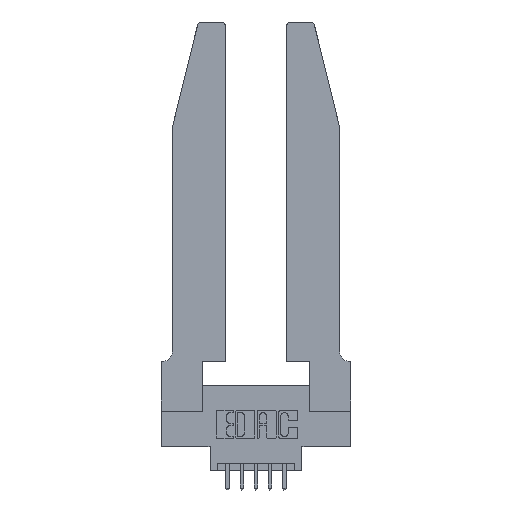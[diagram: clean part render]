
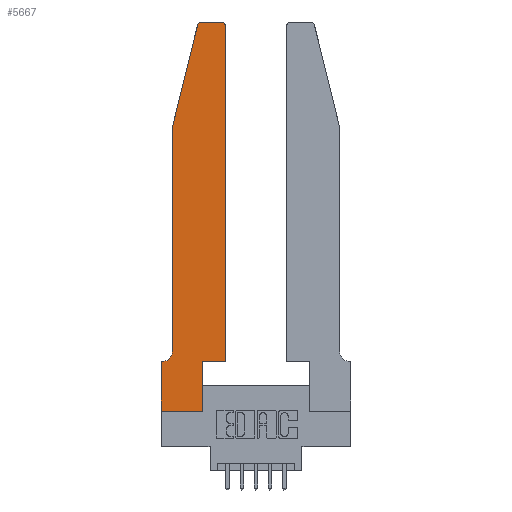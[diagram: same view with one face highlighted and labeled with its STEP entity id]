
A CAD part, top view. The second image highlights one B-rep face of the part: STEP entity #5667.
In plain terms, the highlighted planar face has unit normal (0, 0, 1).
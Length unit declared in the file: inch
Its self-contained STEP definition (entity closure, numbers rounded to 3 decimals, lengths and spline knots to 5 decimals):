
#4 = DIRECTION ( 'NONE',  ( 1., 0., 0. ) ) ;
#141 = VECTOR ( 'NONE', #9166, 39.37008 ) ;
#238 = LINE ( 'NONE', #2902, #11358 ) ;
#588 = CARTESIAN_POINT ( 'NONE',  ( 0.0755, 0.35, 0.37 ) ) ;
#594 = ORIENTED_EDGE ( 'NONE', *, *, #11141, .T. ) ;
#834 = DIRECTION ( 'NONE',  ( -1., 0., 0. ) ) ;
#885 = VERTEX_POINT ( 'NONE', #13201 ) ;
#962 = ORIENTED_EDGE ( 'NONE', *, *, #2790, .T. ) ;
#1181 = AXIS2_PLACEMENT_3D ( 'NONE', #13568, #7385, #834 ) ;
#1326 = DIRECTION ( 'NONE',  ( 0., 0., 1. ) ) ;
#1408 = ORIENTED_EDGE ( 'NONE', *, *, #4355, .T. ) ;
#1425 = DIRECTION ( 'NONE',  ( 0., -1., 0. ) ) ;
#1457 = LINE ( 'NONE', #11783, #10041 ) ;
#1467 = CARTESIAN_POINT ( 'NONE',  ( 0.0755, 2., 0.37 ) ) ;
#1706 = DIRECTION ( 'NONE',  ( 1., 0., 0. ) ) ;
#1748 = CARTESIAN_POINT ( 'NONE',  ( 0.2865, 0.35, 0.37 ) ) ;
#1940 = VECTOR ( 'NONE', #13599, 39.37008 ) ;
#2302 = ORIENTED_EDGE ( 'NONE', *, *, #7899, .T. ) ;
#2636 = ORIENTED_EDGE ( 'NONE', *, *, #11232, .T. ) ;
#2716 = EDGE_LOOP ( 'NONE', ( #1408, #4652, #2302, #10080, #2636, #594, #962, #4663, #4332, #12566, #7375, #9206 ) ) ;
#2720 = CARTESIAN_POINT ( 'NONE',  ( 0., 0., 0.37 ) ) ;
#2774 = VERTEX_POINT ( 'NONE', #11372 ) ;
#2790 = EDGE_CURVE ( 'NONE', #885, #5018, #6215, .T. ) ;
#2902 = CARTESIAN_POINT ( 'NONE',  ( 0.0755, 2., 0.37 ) ) ;
#3075 = LINE ( 'NONE', #5925, #141 ) ;
#3227 = VERTEX_POINT ( 'NONE', #7248 ) ;
#3809 = CIRCLE ( 'NONE', #10134, 0.03 ) ;
#3815 = EDGE_CURVE ( 'NONE', #9651, #10955, #12226, .T. ) ;
#3924 = DIRECTION ( 'NONE',  ( -1., 0., 0. ) ) ;
#4332 = ORIENTED_EDGE ( 'NONE', *, *, #12507, .T. ) ;
#4355 = EDGE_CURVE ( 'NONE', #10137, #9304, #3075, .T. ) ;
#4362 = CARTESIAN_POINT ( 'NONE',  ( 0.2865, 0., 0.37 ) ) ;
#4652 = ORIENTED_EDGE ( 'NONE', *, *, #13527, .T. ) ;
#4663 = ORIENTED_EDGE ( 'NONE', *, *, #12418, .T. ) ;
#4891 = VECTOR ( 'NONE', #3924, 39.37008 ) ;
#4986 = CIRCLE ( 'NONE', #6332, 0.03 ) ;
#5018 = VERTEX_POINT ( 'NONE', #2720 ) ;
#5087 = DIRECTION ( 'NONE',  ( 1., 0., 0. ) ) ;
#5465 = DIRECTION ( 'NONE',  ( 0., 1., 0. ) ) ;
#5641 = VERTEX_POINT ( 'NONE', #11292 ) ;
#5667 = ADVANCED_FACE ( 'NONE', ( #5974 ), #13345, .T. ) ;
#5925 = CARTESIAN_POINT ( 'NONE',  ( 0.2605, 2.75, 0.37 ) ) ;
#5974 = FACE_OUTER_BOUND ( 'NONE', #2716, .T. ) ;
#6215 = LINE ( 'NONE', #11280, #11470 ) ;
#6226 = LINE ( 'NONE', #10391, #8732 ) ;
#6332 = AXIS2_PLACEMENT_3D ( 'NONE', #7872, #1326, #8909 ) ;
#6341 = CARTESIAN_POINT ( 'NONE',  ( 0.2865, 0.35, 0.37 ) ) ;
#6353 = DIRECTION ( 'NONE',  ( 0., 0., 1. ) ) ;
#6500 = AXIS2_PLACEMENT_3D ( 'NONE', #7137, #8232, #1706 ) ;
#6786 = CIRCLE ( 'NONE', #1181, 0.07 ) ;
#7137 = CARTESIAN_POINT ( 'NONE',  ( 0., 0.35, 0.37 ) ) ;
#7248 = CARTESIAN_POINT ( 'NONE',  ( 0.0055, 0.35, 0.37 ) ) ;
#7375 = ORIENTED_EDGE ( 'NONE', *, *, #11894, .T. ) ;
#7385 = DIRECTION ( 'NONE',  ( 0., 0., -1. ) ) ;
#7695 = CARTESIAN_POINT ( 'NONE',  ( 0.4505, 0.35, 0.37 ) ) ;
#7797 = LINE ( 'NONE', #588, #4891 ) ;
#7872 = CARTESIAN_POINT ( 'NONE',  ( 0.4205, 2.72, 0.37 ) ) ;
#7899 = EDGE_CURVE ( 'NONE', #11291, #9651, #238, .T. ) ;
#7977 = CARTESIAN_POINT ( 'NONE',  ( 0.0755, 0.42, 0.37 ) ) ;
#8232 = DIRECTION ( 'NONE',  ( 0., 0., 1. ) ) ;
#8371 = VERTEX_POINT ( 'NONE', #1748 ) ;
#8732 = VECTOR ( 'NONE', #5087, 39.37008 ) ;
#8909 = DIRECTION ( 'NONE',  ( 1., 0., 0. ) ) ;
#9166 = DIRECTION ( 'NONE',  ( -1., 0., 0. ) ) ;
#9206 = ORIENTED_EDGE ( 'NONE', *, *, #13704, .T. ) ;
#9304 = VERTEX_POINT ( 'NONE', #9733 ) ;
#9651 = VERTEX_POINT ( 'NONE', #9866 ) ;
#9733 = CARTESIAN_POINT ( 'NONE',  ( 0.284, 2.75, 0.37 ) ) ;
#9866 = CARTESIAN_POINT ( 'NONE',  ( 0.0755, 2., 0.37 ) ) ;
#10041 = VECTOR ( 'NONE', #5465, 39.37008 ) ;
#10080 = ORIENTED_EDGE ( 'NONE', *, *, #3815, .T. ) ;
#10134 = AXIS2_PLACEMENT_3D ( 'NONE', #12602, #6353, #13615 ) ;
#10137 = VERTEX_POINT ( 'NONE', #13689 ) ;
#10151 = VECTOR ( 'NONE', #1425, 39.37008 ) ;
#10391 = CARTESIAN_POINT ( 'NONE',  ( 0., 0., 0.37 ) ) ;
#10578 = CARTESIAN_POINT ( 'NONE',  ( 0.25487, 2.72718, 0.37 ) ) ;
#10760 = VERTEX_POINT ( 'NONE', #4362 ) ;
#10827 = EDGE_CURVE ( 'NONE', #8371, #5641, #11812, .T. ) ;
#10955 = VERTEX_POINT ( 'NONE', #7977 ) ;
#11141 = EDGE_CURVE ( 'NONE', #3227, #885, #7797, .T. ) ;
#11232 = EDGE_CURVE ( 'NONE', #10955, #3227, #6786, .T. ) ;
#11246 = DIRECTION ( 'NONE',  ( 0., -1., 0. ) ) ;
#11280 = CARTESIAN_POINT ( 'NONE',  ( 0., 0., 0.37 ) ) ;
#11291 = VERTEX_POINT ( 'NONE', #10578 ) ;
#11292 = CARTESIAN_POINT ( 'NONE',  ( 0.4505, 0.35, 0.37 ) ) ;
#11358 = VECTOR ( 'NONE', #13476, 39.37008 ) ;
#11372 = CARTESIAN_POINT ( 'NONE',  ( 0.4505, 2.72, 0.37 ) ) ;
#11470 = VECTOR ( 'NONE', #11246, 39.37008 ) ;
#11500 = VECTOR ( 'NONE', #4, 39.37008 ) ;
#11783 = CARTESIAN_POINT ( 'NONE',  ( 0.4505, 0.35, 0.37 ) ) ;
#11812 = LINE ( 'NONE', #7695, #11500 ) ;
#11894 = EDGE_CURVE ( 'NONE', #5641, #2774, #1457, .T. ) ;
#12226 = LINE ( 'NONE', #1467, #10151 ) ;
#12418 = EDGE_CURVE ( 'NONE', #5018, #10760, #6226, .T. ) ;
#12507 = EDGE_CURVE ( 'NONE', #10760, #8371, #13236, .T. ) ;
#12566 = ORIENTED_EDGE ( 'NONE', *, *, #10827, .T. ) ;
#12602 = CARTESIAN_POINT ( 'NONE',  ( 0.284, 2.72, 0.37 ) ) ;
#13201 = CARTESIAN_POINT ( 'NONE',  ( 0., 0.35, 0.37 ) ) ;
#13236 = LINE ( 'NONE', #6341, #1940 ) ;
#13345 = PLANE ( 'NONE',  #6500 ) ;
#13476 = DIRECTION ( 'NONE',  ( -0.239, -0.971, 0. ) ) ;
#13527 = EDGE_CURVE ( 'NONE', #9304, #11291, #3809, .T. ) ;
#13568 = CARTESIAN_POINT ( 'NONE',  ( 0.0055, 0.42, 0.37 ) ) ;
#13599 = DIRECTION ( 'NONE',  ( 0., 1., 0. ) ) ;
#13615 = DIRECTION ( 'NONE',  ( 1., 0., 0. ) ) ;
#13689 = CARTESIAN_POINT ( 'NONE',  ( 0.4205, 2.75, 0.37 ) ) ;
#13704 = EDGE_CURVE ( 'NONE', #2774, #10137, #4986, .T. ) ;
